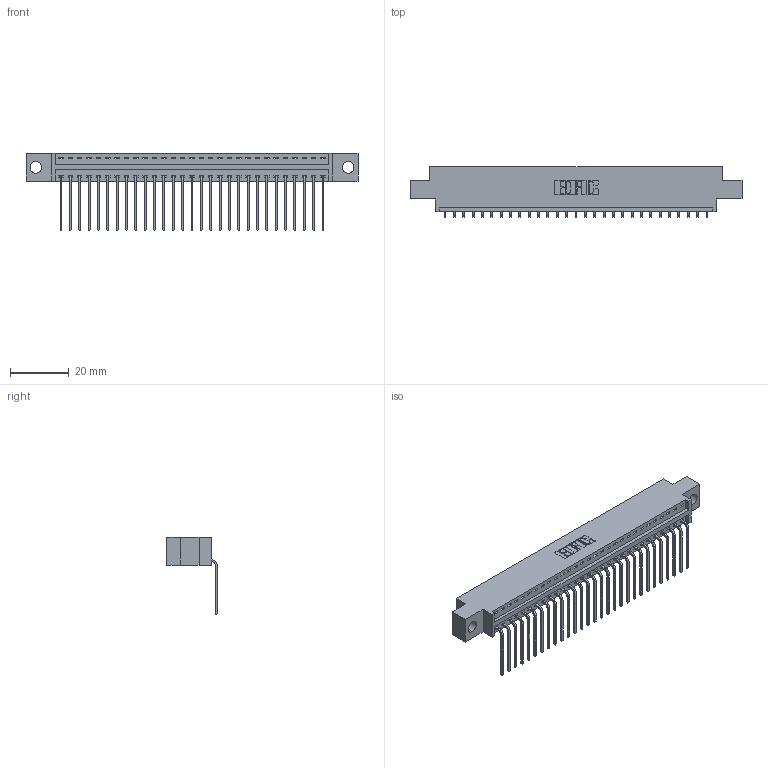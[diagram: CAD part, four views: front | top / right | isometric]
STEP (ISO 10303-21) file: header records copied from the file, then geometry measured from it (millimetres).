
FILE_DESCRIPTION (( 'STEP AP203' ), '1' );
FILE_NAME ('346-029-559-604.STEP', '2022-05-06T15:04:54', ( '' ), ( '' ), 'SwSTEP 2.0', 'SolidWorks 2020', '' );
FILE_SCHEMA (( 'CONFIG_CONTROL_DESIGN' ));
Length unit declared in the file: inch
Products named in the file (3): 346-029-559-604; 345-292-001_558 559 Tail - 1; 346 Part_0.170 Offset - 0.156 Dia-TH
Assembly tree (30 placements, depth 2):
  346-029-559-604
    346 Part_0.170 Offset - 0.156 Dia-TH
    345-292-001_558 559 Tail - 1  x29
Bounding box: 112.65 x 17.08 x 26.16 mm (x, y, z)
Volume: 10529.5 mm3; surface area: 13594.2 mm2
Topology: 30 solids, 30 shells, 1880 faces, 5655 edges, 3730 vertices
Faces by surface type: plane 1312, cylinder 568
Entity records: 20383 total; most frequent: CARTESIAN_POINT 3509, ORIENTED_EDGE 3470, DIRECTION 3109, EDGE_CURVE 1735, VECTOR 1487, LINE 1487, VERTEX_POINT 1154, AXIS2_PLACEMENT_3D 811
